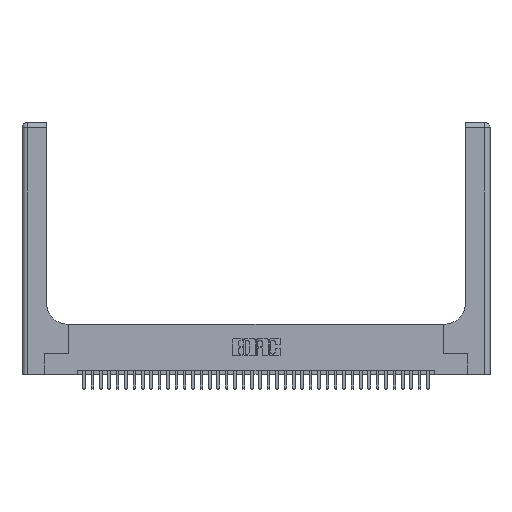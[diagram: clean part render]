
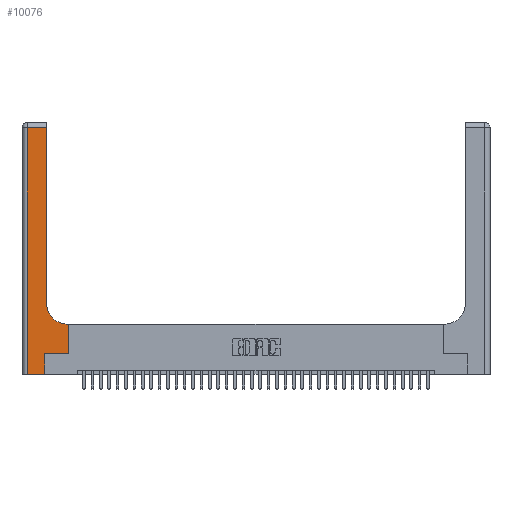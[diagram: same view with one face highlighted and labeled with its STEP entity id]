
A CAD part, top view. The second image highlights one B-rep face of the part: STEP entity #10076.
In plain terms, the highlighted planar face has unit normal (0, 0, 1).
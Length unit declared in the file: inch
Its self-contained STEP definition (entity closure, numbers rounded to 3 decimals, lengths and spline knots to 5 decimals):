
#78 = CARTESIAN_POINT ( 'NONE',  ( 0.5415, 0.6, 0.37 ) ) ;
#612 = CARTESIAN_POINT ( 'NONE',  ( 0., 2.94, 0.37 ) ) ;
#721 = DIRECTION ( 'NONE',  ( 1., 0., 0. ) ) ;
#986 = VERTEX_POINT ( 'NONE', #9775 ) ;
#1217 = ORIENTED_EDGE ( 'NONE', *, *, #32461, .T. ) ;
#1362 = CARTESIAN_POINT ( 'NONE',  ( 0.269, 0.25, 0.37 ) ) ;
#2010 = VERTEX_POINT ( 'NONE', #78 ) ;
#2805 = LINE ( 'NONE', #9468, #26440 ) ;
#2885 = VERTEX_POINT ( 'NONE', #30536 ) ;
#3141 = ORIENTED_EDGE ( 'NONE', *, *, #21832, .T. ) ;
#4983 = LINE ( 'NONE', #28525, #20742 ) ;
#5827 = DIRECTION ( 'NONE',  ( 0., 1., 0. ) ) ;
#6703 = DIRECTION ( 'NONE',  ( -1., 0., 0. ) ) ;
#7387 = VECTOR ( 'NONE', #22215, 39.37008 ) ;
#7431 = EDGE_CURVE ( 'NONE', #2010, #9231, #24335, .T. ) ;
#8278 = CARTESIAN_POINT ( 'NONE',  ( 0.2915, 2.94, 0.37 ) ) ;
#8579 = ORIENTED_EDGE ( 'NONE', *, *, #7431, .T. ) ;
#9004 = VERTEX_POINT ( 'NONE', #22570 ) ;
#9185 = CARTESIAN_POINT ( 'NONE',  ( 0.269, 0., 0.37 ) ) ;
#9231 = VERTEX_POINT ( 'NONE', #17642 ) ;
#9459 = DIRECTION ( 'NONE',  ( 0., 1., 0. ) ) ;
#9468 = CARTESIAN_POINT ( 'NONE',  ( 0.06, 3., 0.37 ) ) ;
#9775 = CARTESIAN_POINT ( 'NONE',  ( 0.06, 2.94, 0.37 ) ) ;
#10002 = VECTOR ( 'NONE', #34489, 39.37008 ) ;
#10076 = ADVANCED_FACE ( 'NONE', ( #13538 ), #18480, .F. ) ;
#10927 = LINE ( 'NONE', #19752, #10002 ) ;
#12200 = ORIENTED_EDGE ( 'NONE', *, *, #24525, .T. ) ;
#12712 = DIRECTION ( 'NONE',  ( -1., 0., 0. ) ) ;
#13272 = VERTEX_POINT ( 'NONE', #13906 ) ;
#13538 = FACE_OUTER_BOUND ( 'NONE', #37552, .T. ) ;
#13906 = CARTESIAN_POINT ( 'NONE',  ( 0.269, 0.25, 0.37 ) ) ;
#14942 = ORIENTED_EDGE ( 'NONE', *, *, #28070, .T. ) ;
#15601 = ORIENTED_EDGE ( 'NONE', *, *, #21803, .T. ) ;
#15709 = AXIS2_PLACEMENT_3D ( 'NONE', #21458, #24403, #6703 ) ;
#16545 = ORIENTED_EDGE ( 'NONE', *, *, #25155, .T. ) ;
#17642 = CARTESIAN_POINT ( 'NONE',  ( 0.2915, 0.85, 0.37 ) ) ;
#17808 = VECTOR ( 'NONE', #9459, 39.37008 ) ;
#18480 = PLANE ( 'NONE',  #15709 ) ;
#18606 = DIRECTION ( 'NONE',  ( 0., 0., -1. ) ) ;
#18994 = VECTOR ( 'NONE', #12712, 39.37008 ) ;
#19752 = CARTESIAN_POINT ( 'NONE',  ( 0.2915, 0.6, 0.37 ) ) ;
#19800 = LINE ( 'NONE', #25561, #34478 ) ;
#20414 = LINE ( 'NONE', #20598, #35059 ) ;
#20598 = CARTESIAN_POINT ( 'NONE',  ( 0.269, 0., 0.37 ) ) ;
#20742 = VECTOR ( 'NONE', #28402, 39.37008 ) ;
#21458 = CARTESIAN_POINT ( 'NONE',  ( 0., 3., 0.37 ) ) ;
#21803 = EDGE_CURVE ( 'NONE', #2885, #26211, #4983, .T. ) ;
#21832 = EDGE_CURVE ( 'NONE', #9004, #29082, #19800, .T. ) ;
#22215 = DIRECTION ( 'NONE',  ( 1., 0., 0. ) ) ;
#22570 = CARTESIAN_POINT ( 'NONE',  ( 0.5585, 0.25, 0.37 ) ) ;
#24279 = EDGE_CURVE ( 'NONE', #26211, #13272, #20414, .T. ) ;
#24335 = CIRCLE ( 'NONE', #36362, 0.25 ) ;
#24403 = DIRECTION ( 'NONE',  ( 0., 0., -1. ) ) ;
#24439 = CARTESIAN_POINT ( 'NONE',  ( 0.5585, 0.6, 0.37 ) ) ;
#24525 = EDGE_CURVE ( 'NONE', #34384, #986, #26818, .T. ) ;
#25155 = EDGE_CURVE ( 'NONE', #13272, #9004, #37696, .T. ) ;
#25561 = CARTESIAN_POINT ( 'NONE',  ( 0.5585, 0.25, 0.37 ) ) ;
#25615 = LINE ( 'NONE', #35812, #17808 ) ;
#26211 = VERTEX_POINT ( 'NONE', #9185 ) ;
#26440 = VECTOR ( 'NONE', #30089, 39.37008 ) ;
#26818 = LINE ( 'NONE', #612, #18994 ) ;
#28070 = EDGE_CURVE ( 'NONE', #29082, #2010, #10927, .T. ) ;
#28402 = DIRECTION ( 'NONE',  ( 1., 0., 0. ) ) ;
#28525 = CARTESIAN_POINT ( 'NONE',  ( 0., 0., 0.37 ) ) ;
#29019 = EDGE_CURVE ( 'NONE', #9231, #34384, #25615, .T. ) ;
#29082 = VERTEX_POINT ( 'NONE', #24439 ) ;
#30089 = DIRECTION ( 'NONE',  ( 0., -1., 0. ) ) ;
#30536 = CARTESIAN_POINT ( 'NONE',  ( 0.06, 0., 0.37 ) ) ;
#31446 = ORIENTED_EDGE ( 'NONE', *, *, #24279, .T. ) ;
#32461 = EDGE_CURVE ( 'NONE', #986, #2885, #2805, .T. ) ;
#33737 = ORIENTED_EDGE ( 'NONE', *, *, #29019, .T. ) ;
#34384 = VERTEX_POINT ( 'NONE', #8278 ) ;
#34478 = VECTOR ( 'NONE', #37297, 39.37008 ) ;
#34489 = DIRECTION ( 'NONE',  ( -1., 0., 0. ) ) ;
#35059 = VECTOR ( 'NONE', #5827, 39.37008 ) ;
#35812 = CARTESIAN_POINT ( 'NONE',  ( 0.2915, 3., 0.37 ) ) ;
#36161 = CARTESIAN_POINT ( 'NONE',  ( 0.5415, 0.85, 0.37 ) ) ;
#36362 = AXIS2_PLACEMENT_3D ( 'NONE', #36161, #18606, #721 ) ;
#37297 = DIRECTION ( 'NONE',  ( 0., 1., 0. ) ) ;
#37552 = EDGE_LOOP ( 'NONE', ( #33737, #12200, #1217, #15601, #31446, #16545, #3141, #14942, #8579 ) ) ;
#37696 = LINE ( 'NONE', #1362, #7387 ) ;
